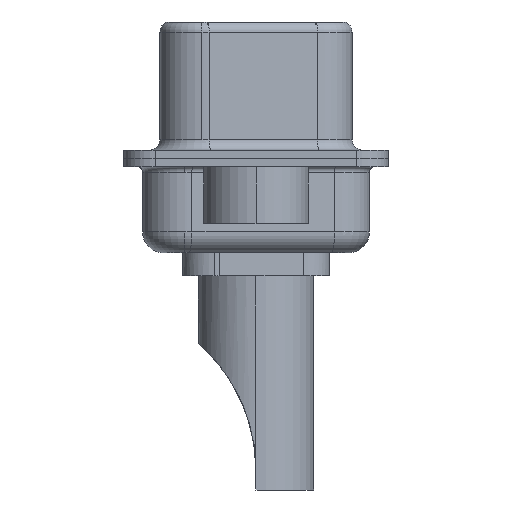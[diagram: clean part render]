
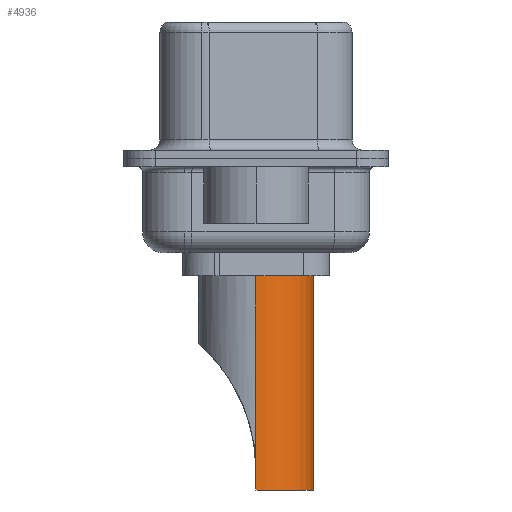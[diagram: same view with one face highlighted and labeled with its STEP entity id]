
A CAD part, left-side view. The second image highlights one B-rep face of the part: STEP entity #4936.
In plain terms, the highlighted cylindrical face has radius 2.75 mm (diameter 5.5 mm), a partial arc.
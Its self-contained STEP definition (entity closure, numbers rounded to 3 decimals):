
#336 = VECTOR ( 'NONE', #10965, 1000. ) ;
#546 = VERTEX_POINT ( 'NONE', #9801 ) ;
#1648 = EDGE_CURVE ( 'NONE', #5157, #21794, #7835, .T. ) ;
#2827 = AXIS2_PLACEMENT_3D ( 'NONE', #12398, #6699, #15112 ) ;
#2829 = EDGE_CURVE ( 'NONE', #4502, #5036, #15499, .T. ) ;
#3046 = EDGE_CURVE ( 'NONE', #20832, #21794, #10590, .T. ) ;
#3069 = CYLINDRICAL_SURFACE ( 'NONE', #2827, 2.75 ) ;
#4162 = EDGE_CURVE ( 'NONE', #4502, #5157, #21673, .T. ) ;
#4502 = VERTEX_POINT ( 'NONE', #16323 ) ;
#4936 = ADVANCED_FACE ( 'NONE', ( #13194 ), #3069, .T. ) ;
#5036 = VERTEX_POINT ( 'NONE', #21940 ) ;
#5157 = VERTEX_POINT ( 'NONE', #15670 ) ;
#5252 = VECTOR ( 'NONE', #22445, 1000. ) ;
#5542 = VECTOR ( 'NONE', #23046, 1000. ) ;
#6386 = DIRECTION ( 'NONE',  ( 1., 0., 0. ) ) ;
#6419 = DIRECTION ( 'NONE',  ( 0., 0., 1. ) ) ;
#6548 = CARTESIAN_POINT ( 'NONE',  ( 0., 0., 1.5 ) ) ;
#6699 = DIRECTION ( 'NONE',  ( 0., 0., 1. ) ) ;
#7835 = CIRCLE ( 'NONE', #21601, 2.75 ) ;
#8460 = DIRECTION ( 'NONE',  ( 1., 0., 0. ) ) ;
#9308 = CARTESIAN_POINT ( 'NONE',  ( 2.75, 0., 4.234 ) ) ;
#9700 = LINE ( 'NONE', #9308, #5252 ) ;
#9801 = CARTESIAN_POINT ( 'NONE',  ( 2.75, 0., 1.5 ) ) ;
#9923 = CARTESIAN_POINT ( 'NONE',  ( -2.75, 0., 4.234 ) ) ;
#10036 = CARTESIAN_POINT ( 'NONE',  ( 2.75, 0., -8.7 ) ) ;
#10590 = LINE ( 'NONE', #24323, #5542 ) ;
#10916 = ORIENTED_EDGE ( 'NONE', *, *, #1648, .T. ) ;
#10965 = DIRECTION ( 'NONE',  ( 0., 0., 1. ) ) ;
#11075 = ORIENTED_EDGE ( 'NONE', *, *, #23378, .T. ) ;
#11631 = ORIENTED_EDGE ( 'NONE', *, *, #17507, .F. ) ;
#12398 = CARTESIAN_POINT ( 'NONE',  ( 0., 0., 4.234 ) ) ;
#12423 = ORIENTED_EDGE ( 'NONE', *, *, #3046, .F. ) ;
#13118 = EDGE_LOOP ( 'NONE', ( #14949, #22050, #10916, #12423, #11075, #11631 ) ) ;
#13194 = FACE_OUTER_BOUND ( 'NONE', #13118, .T. ) ;
#14092 = CIRCLE ( 'NONE', #23812, 2.75 ) ;
#14949 = ORIENTED_EDGE ( 'NONE', *, *, #2829, .F. ) ;
#15112 = DIRECTION ( 'NONE',  ( 1., 0., 0. ) ) ;
#15499 = LINE ( 'NONE', #9923, #336 ) ;
#15670 = CARTESIAN_POINT ( 'NONE',  ( -2.75, 0., -8.7 ) ) ;
#16323 = CARTESIAN_POINT ( 'NONE',  ( -2.75, 0., -7.764 ) ) ;
#16723 = VECTOR ( 'NONE', #18249, 1000. ) ;
#16769 = CARTESIAN_POINT ( 'NONE',  ( 2.75, 0., -7.764 ) ) ;
#17507 = EDGE_CURVE ( 'NONE', #5036, #546, #14092, .T. ) ;
#18034 = CARTESIAN_POINT ( 'NONE',  ( 0., 0., -8.7 ) ) ;
#18249 = DIRECTION ( 'NONE',  ( 0., 0., -1. ) ) ;
#19625 = CARTESIAN_POINT ( 'NONE',  ( -2.75, 0., -8.7 ) ) ;
#19761 = DIRECTION ( 'NONE',  ( 0., 0., 1. ) ) ;
#20832 = VERTEX_POINT ( 'NONE', #16769 ) ;
#21601 = AXIS2_PLACEMENT_3D ( 'NONE', #18034, #6419, #6386 ) ;
#21673 = LINE ( 'NONE', #19625, #16723 ) ;
#21794 = VERTEX_POINT ( 'NONE', #10036 ) ;
#21940 = CARTESIAN_POINT ( 'NONE',  ( -2.75, 0., 1.5 ) ) ;
#22050 = ORIENTED_EDGE ( 'NONE', *, *, #4162, .T. ) ;
#22445 = DIRECTION ( 'NONE',  ( 0., 0., 1. ) ) ;
#23046 = DIRECTION ( 'NONE',  ( 0., 0., -1. ) ) ;
#23378 = EDGE_CURVE ( 'NONE', #20832, #546, #9700, .T. ) ;
#23812 = AXIS2_PLACEMENT_3D ( 'NONE', #6548, #19761, #8460 ) ;
#24323 = CARTESIAN_POINT ( 'NONE',  ( 2.75, 0., -8.7 ) ) ;
